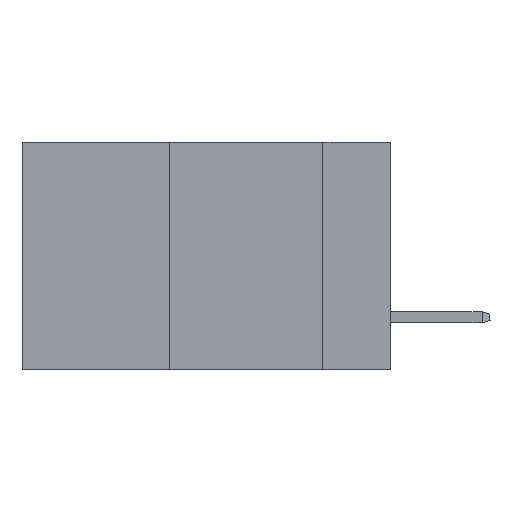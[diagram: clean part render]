
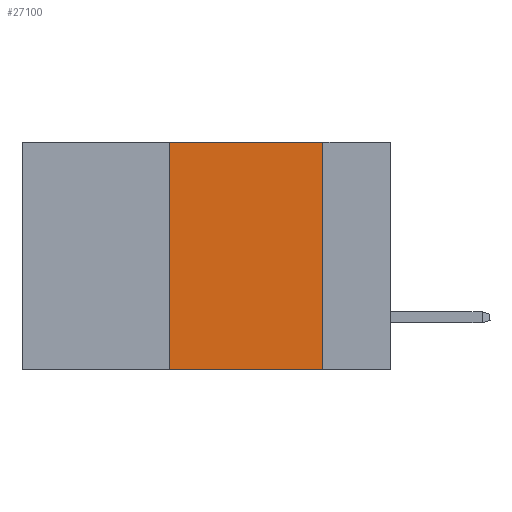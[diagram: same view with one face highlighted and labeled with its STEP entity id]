
A CAD part, left-side view. The second image highlights one B-rep face of the part: STEP entity #27100.
In plain terms, the highlighted planar face has unit normal (-1, 0, 0).
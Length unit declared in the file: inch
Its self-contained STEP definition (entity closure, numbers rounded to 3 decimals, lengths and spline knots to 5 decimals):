
#548 = DIRECTION ( 'NONE',  ( 0., 0., 1. ) ) ;
#1123 = ORIENTED_EDGE ( 'NONE', *, *, #4521, .F. ) ;
#2532 = LINE ( 'NONE', #15064, #21383 ) ;
#2792 = LINE ( 'NONE', #5475, #12971 ) ;
#2795 = PLANE ( 'NONE',  #5289 ) ;
#3745 = LINE ( 'NONE', #10619, #22602 ) ;
#4521 = EDGE_CURVE ( 'NONE', #22260, #19002, #3745, .T. ) ;
#4728 = DIRECTION ( 'NONE',  ( 0., -1., 0. ) ) ;
#4896 = CARTESIAN_POINT ( 'NONE',  ( 0., 0.6, 0. ) ) ;
#5171 = DIRECTION ( 'NONE',  ( 1., 0., 0. ) ) ;
#5289 = AXIS2_PLACEMENT_3D ( 'NONE', #4896, #5171, #7234 ) ;
#5475 = CARTESIAN_POINT ( 'NONE',  ( 0., 0.6, 0. ) ) ;
#7234 = DIRECTION ( 'NONE',  ( 0., 0., -1. ) ) ;
#7236 = EDGE_CURVE ( 'NONE', #23472, #14085, #25335, .T. ) ;
#7265 = FACE_OUTER_BOUND ( 'NONE', #19684, .T. ) ;
#8040 = ORIENTED_EDGE ( 'NONE', *, *, #7236, .F. ) ;
#9319 = ORIENTED_EDGE ( 'NONE', *, *, #16329, .T. ) ;
#10619 = CARTESIAN_POINT ( 'NONE',  ( 0., 0.11, 0. ) ) ;
#11828 = DIRECTION ( 'NONE',  ( 0., -1., 0. ) ) ;
#12379 = VECTOR ( 'NONE', #548, 39.37008 ) ;
#12971 = VECTOR ( 'NONE', #11828, 39.37008 ) ;
#13399 = CARTESIAN_POINT ( 'NONE',  ( 0., 0.11, 0. ) ) ;
#14085 = VERTEX_POINT ( 'NONE', #19378 ) ;
#14693 = DIRECTION ( 'NONE',  ( 0., 0., -1. ) ) ;
#15064 = CARTESIAN_POINT ( 'NONE',  ( 0., 0.6, -0.37 ) ) ;
#16329 = EDGE_CURVE ( 'NONE', #23472, #19002, #2532, .T. ) ;
#19002 = VERTEX_POINT ( 'NONE', #22202 ) ;
#19378 = CARTESIAN_POINT ( 'NONE',  ( 0., 0.36, 0. ) ) ;
#19684 = EDGE_LOOP ( 'NONE', ( #1123, #23137, #8040, #9319 ) ) ;
#21383 = VECTOR ( 'NONE', #4728, 39.37008 ) ;
#22202 = CARTESIAN_POINT ( 'NONE',  ( 0., 0.11, -0.37 ) ) ;
#22260 = VERTEX_POINT ( 'NONE', #13399 ) ;
#22602 = VECTOR ( 'NONE', #14693, 39.37008 ) ;
#23137 = ORIENTED_EDGE ( 'NONE', *, *, #24133, .F. ) ;
#23472 = VERTEX_POINT ( 'NONE', #24294 ) ;
#24133 = EDGE_CURVE ( 'NONE', #14085, #22260, #2792, .T. ) ;
#24294 = CARTESIAN_POINT ( 'NONE',  ( 0., 0.36, -0.37 ) ) ;
#25335 = LINE ( 'NONE', #25811, #12379 ) ;
#25811 = CARTESIAN_POINT ( 'NONE',  ( 0., 0.36, 0. ) ) ;
#27100 = ADVANCED_FACE ( 'NONE', ( #7265 ), #2795, .F. ) ;
